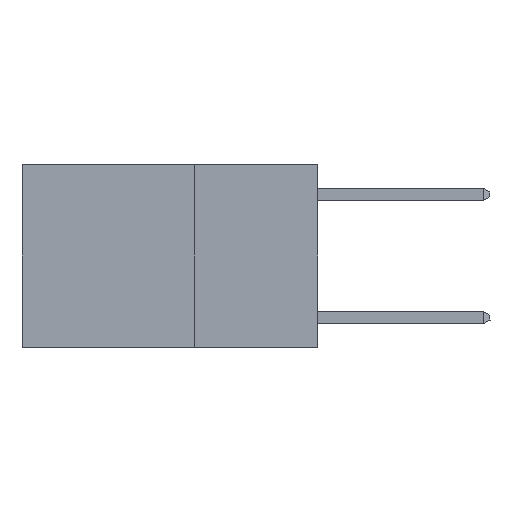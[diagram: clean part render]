
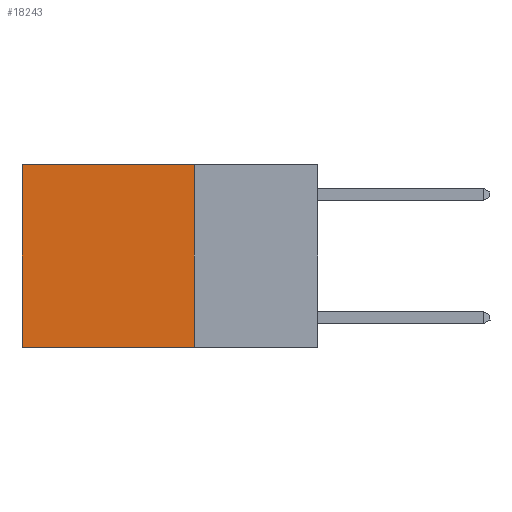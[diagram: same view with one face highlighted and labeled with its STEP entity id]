
A CAD part, left-side view. The second image highlights one B-rep face of the part: STEP entity #18243.
In plain terms, the highlighted planar face has unit normal (-1, 0, 0).
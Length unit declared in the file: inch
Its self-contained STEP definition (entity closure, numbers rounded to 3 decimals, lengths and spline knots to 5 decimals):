
#75 = ORIENTED_EDGE ( 'NONE', *, *, #16223, .T. ) ;
#398 = LINE ( 'NONE', #18188, #19267 ) ;
#591 = VERTEX_POINT ( 'NONE', #4161 ) ;
#1474 = LINE ( 'NONE', #5177, #19723 ) ;
#1536 = CARTESIAN_POINT ( 'NONE',  ( 0.2625, 0.6, 0. ) ) ;
#3260 = VERTEX_POINT ( 'NONE', #4337 ) ;
#3387 = VECTOR ( 'NONE', #21093, 39.37008 ) ;
#3707 = ORIENTED_EDGE ( 'NONE', *, *, #9797, .F. ) ;
#4149 = EDGE_CURVE ( 'NONE', #20731, #18372, #1474, .T. ) ;
#4161 = CARTESIAN_POINT ( 'NONE',  ( 0.2625, 0.25, 0. ) ) ;
#4337 = CARTESIAN_POINT ( 'NONE',  ( 0.2625, 0.25, -0.37 ) ) ;
#5177 = CARTESIAN_POINT ( 'NONE',  ( 0.2625, 0.6, 0. ) ) ;
#6885 = EDGE_CURVE ( 'NONE', #3260, #18372, #21477, .T. ) ;
#7007 = DIRECTION ( 'NONE',  ( 0., 0., -1. ) ) ;
#7073 = LINE ( 'NONE', #12153, #15895 ) ;
#8214 = CARTESIAN_POINT ( 'NONE',  ( 0.2625, 0.25, 0. ) ) ;
#8965 = CARTESIAN_POINT ( 'NONE',  ( 0.2625, 0.25, -0.37 ) ) ;
#9035 = ORIENTED_EDGE ( 'NONE', *, *, #4149, .T. ) ;
#9556 = AXIS2_PLACEMENT_3D ( 'NONE', #8214, #20378, #10010 ) ;
#9797 = EDGE_CURVE ( 'NONE', #591, #3260, #398, .T. ) ;
#10010 = DIRECTION ( 'NONE',  ( 0., 0., -1. ) ) ;
#11222 = FACE_OUTER_BOUND ( 'NONE', #13023, .T. ) ;
#12153 = CARTESIAN_POINT ( 'NONE',  ( 0.2625, 0.25, 0. ) ) ;
#13023 = EDGE_LOOP ( 'NONE', ( #9035, #13740, #3707, #75 ) ) ;
#13740 = ORIENTED_EDGE ( 'NONE', *, *, #6885, .F. ) ;
#13900 = DIRECTION ( 'NONE',  ( 0., 1., 0. ) ) ;
#15895 = VECTOR ( 'NONE', #13900, 39.37008 ) ;
#16223 = EDGE_CURVE ( 'NONE', #591, #20731, #7073, .T. ) ;
#18188 = CARTESIAN_POINT ( 'NONE',  ( 0.2625, 0.25, 0. ) ) ;
#18243 = ADVANCED_FACE ( 'NONE', ( #11222 ), #18716, .F. ) ;
#18372 = VERTEX_POINT ( 'NONE', #19005 ) ;
#18716 = PLANE ( 'NONE',  #9556 ) ;
#19005 = CARTESIAN_POINT ( 'NONE',  ( 0.2625, 0.6, -0.37 ) ) ;
#19267 = VECTOR ( 'NONE', #19787, 39.37008 ) ;
#19723 = VECTOR ( 'NONE', #7007, 39.37008 ) ;
#19787 = DIRECTION ( 'NONE',  ( 0., 0., -1. ) ) ;
#20378 = DIRECTION ( 'NONE',  ( 1., 0., 0. ) ) ;
#20731 = VERTEX_POINT ( 'NONE', #1536 ) ;
#21093 = DIRECTION ( 'NONE',  ( 0., 1., 0. ) ) ;
#21477 = LINE ( 'NONE', #8965, #3387 ) ;
